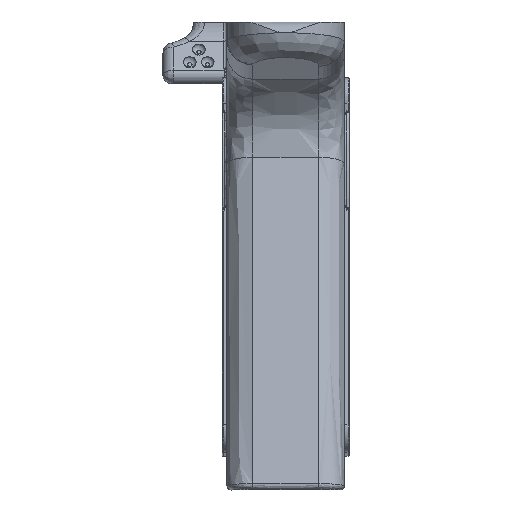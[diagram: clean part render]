
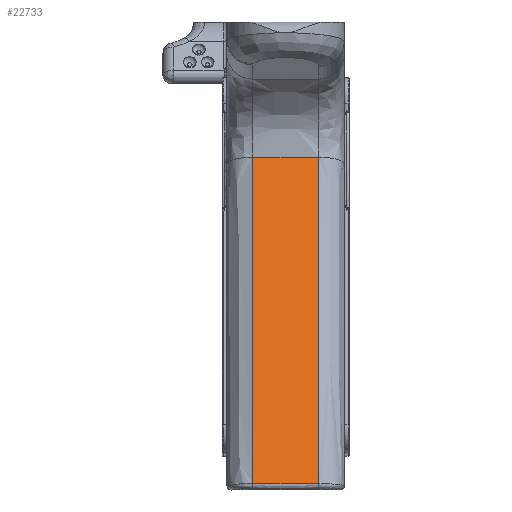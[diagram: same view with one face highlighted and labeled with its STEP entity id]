
A CAD part, front view. The second image highlights one B-rep face of the part: STEP entity #22733.
In plain terms, the highlighted free-form (B-spline) face has degree [5, 1] with [25, 2] control points.
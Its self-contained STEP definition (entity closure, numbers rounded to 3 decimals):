
#752=(
BOUNDED_SURFACE()
B_SPLINE_SURFACE(5,1,((#31762,#31763),(#31764,#31765),(#31766,#31767),(#31768,
#31769),(#31770,#31771),(#31772,#31773),(#31774,#31775),(#31776,#31777),
(#31778,#31779),(#31780,#31781),(#31782,#31783),(#31784,#31785),(#31786,
#31787),(#31788,#31789),(#31790,#31791),(#31792,#31793),(#31794,#31795),
(#31796,#31797),(#31798,#31799),(#31800,#31801),(#31802,#31803),(#31804,
#31805),(#31806,#31807),(#31808,#31809),(#31810,#31811)),.UNSPECIFIED.,
 .F.,.F.,.F.)
B_SPLINE_SURFACE_WITH_KNOTS((6,5,1,1,1,1,1,1,1,1,1,5,6),(2,2),(-1.178,
-1.,-0.9,-0.8,-0.7,-0.6,-0.5,-0.4,-0.3,-0.2,-0.1,0.,2.179),(-2.379,
5.132),.UNSPECIFIED.)
GEOMETRIC_REPRESENTATION_ITEM()
RATIONAL_B_SPLINE_SURFACE(((1.,1.),(1.,1.),(1.,1.),(1.,1.),(1.,1.),(1.,
1.),(1.,1.),(1.,1.),(1.,1.),(1.,1.),(1.,1.),(1.,1.),(1.,1.),(1.,1.),(1.,
1.),(1.,1.),(1.,1.),(1.,1.),(1.,1.),(1.,1.),(1.,1.),(1.,1.),(1.,1.),(1.,
1.),(1.,1.)))
REPRESENTATION_ITEM('')
SURFACE()
);
#1715=B_SPLINE_CURVE_WITH_KNOTS('',3,(#30385,#30386,#30387,#30388,#30389,
#30390),.UNSPECIFIED.,.F.,.F.,(4,2,4),(-7.954,-0.629,
0.),.UNSPECIFIED.);
#1726=B_SPLINE_CURVE_WITH_KNOTS('',3,(#30677,#30678,#30679,#30680,#30681,
#30682,#30683),.UNSPECIFIED.,.F.,.F.,(4,2,1,4),(-7.954,-7.325,
-3.139,0.),.UNSPECIFIED.);
#1804=B_SPLINE_CURVE_WITH_KNOTS('',3,(#31754,#31755,#31756,#31757),
 .UNSPECIFIED.,.F.,.F.,(4,4),(0.6,2.145),.UNSPECIFIED.);
#2730=FACE_OUTER_BOUND('',#4118,.T.);
#4118=EDGE_LOOP('',(#15547,#15548,#15549,#15550));
#5507=LINE('',#30283,#7095);
#7095=VECTOR('',#25575,10.);
#9281=VERTEX_POINT('',#30155);
#9289=VERTEX_POINT('',#30282);
#9291=VERTEX_POINT('',#30384);
#9330=VERTEX_POINT('',#30675);
#11587=EDGE_CURVE('',#9281,#9289,#5507,.T.);
#11591=EDGE_CURVE('',#9289,#9291,#1715,.T.);
#11644=EDGE_CURVE('',#9330,#9281,#1726,.T.);
#11855=EDGE_CURVE('',#9291,#9330,#1804,.T.);
#15547=ORIENTED_EDGE('',*,*,#11591,.F.);
#15548=ORIENTED_EDGE('',*,*,#11587,.F.);
#15549=ORIENTED_EDGE('',*,*,#11644,.F.);
#15550=ORIENTED_EDGE('',*,*,#11855,.F.);
#22733=ADVANCED_FACE('',(#2730),#752,.F.);
#25575=DIRECTION('',(1.,0.,0.));
#30155=CARTESIAN_POINT('',(0.725,-90.162,100.53));
#30282=CARTESIAN_POINT('',(16.175,-90.162,100.53));
#30283=CARTESIAN_POINT('',(22.175,-90.162,100.53));
#30384=CARTESIAN_POINT('',(16.175,-68.765,24.118));
#30385=CARTESIAN_POINT('Ctrl Pts',(16.175,-90.162,100.53));
#30386=CARTESIAN_POINT('Ctrl Pts',(16.175,-83.279,77.132));
#30387=CARTESIAN_POINT('Ctrl Pts',(16.175,-76.502,53.727));
#30388=CARTESIAN_POINT('Ctrl Pts',(16.175,-69.825,28.185));
#30389=CARTESIAN_POINT('Ctrl Pts',(16.175,-69.294,26.148));
#30390=CARTESIAN_POINT('Ctrl Pts',(16.175,-68.765,24.118));
#30675=CARTESIAN_POINT('',(0.725,-68.765,24.118));
#30677=CARTESIAN_POINT('Ctrl Pts',(0.725,-68.765,24.118));
#30678=CARTESIAN_POINT('Ctrl Pts',(0.725,-69.294,
26.148));
#30679=CARTESIAN_POINT('Ctrl Pts',(0.725,-69.824,
28.178));
#30680=CARTESIAN_POINT('Ctrl Pts',(0.725,-73.858,
43.642));
#30681=CARTESIAN_POINT('Ctrl Pts',(0.725,-80.386,
67.092));
#30682=CARTESIAN_POINT('Ctrl Pts',(0.725,-87.212,
90.502));
#30683=CARTESIAN_POINT('Ctrl Pts',(0.725,-90.162,
100.53));
#31754=CARTESIAN_POINT('Ctrl Pts',(16.175,-68.765,24.118));
#31755=CARTESIAN_POINT('Ctrl Pts',(11.025,-68.765,24.118));
#31756=CARTESIAN_POINT('Ctrl Pts',(5.875,-68.765,24.118));
#31757=CARTESIAN_POINT('Ctrl Pts',(0.725,-68.765,24.118));
#31762=CARTESIAN_POINT('Ctrl Pts',(45.968,-95.649,119.15));
#31763=CARTESIAN_POINT('Ctrl Pts',(-29.15,-95.649,
119.15));
#31764=CARTESIAN_POINT('Ctrl Pts',(45.968,-94.719,115.995));
#31765=CARTESIAN_POINT('Ctrl Pts',(-29.15,-94.719,
115.995));
#31766=CARTESIAN_POINT('Ctrl Pts',(45.968,-93.789,112.841));
#31767=CARTESIAN_POINT('Ctrl Pts',(-29.15,-93.789,112.841));
#31768=CARTESIAN_POINT('Ctrl Pts',(45.968,-92.86,109.686));
#31769=CARTESIAN_POINT('Ctrl Pts',(-29.15,-92.86,
109.686));
#31770=CARTESIAN_POINT('Ctrl Pts',(45.968,-91.93,106.531));
#31771=CARTESIAN_POINT('Ctrl Pts',(-29.15,-91.93,
106.531));
#31772=CARTESIAN_POINT('Ctrl Pts',(45.968,-91.,103.376));
#31773=CARTESIAN_POINT('Ctrl Pts',(-29.15,-91.,
103.376));
#31774=CARTESIAN_POINT('Ctrl Pts',(45.968,-90.477,101.6));
#31775=CARTESIAN_POINT('Ctrl Pts',(-29.15,-90.477,
101.6));
#31776=CARTESIAN_POINT('Ctrl Pts',(45.968,-89.439,98.075));
#31777=CARTESIAN_POINT('Ctrl Pts',(-29.15,-89.439,
98.075));
#31778=CARTESIAN_POINT('Ctrl Pts',(45.968,-87.911,92.865));
#31779=CARTESIAN_POINT('Ctrl Pts',(-29.15,-87.911,
92.865));
#31780=CARTESIAN_POINT('Ctrl Pts',(45.968,-85.928,86.075));
#31781=CARTESIAN_POINT('Ctrl Pts',(-29.15,-85.928,
86.075));
#31782=CARTESIAN_POINT('Ctrl Pts',(45.968,-83.55,77.871));
#31783=CARTESIAN_POINT('Ctrl Pts',(-29.15,-83.55,
77.871));
#31784=CARTESIAN_POINT('Ctrl Pts',(45.968,-81.281,69.978));
#31785=CARTESIAN_POINT('Ctrl Pts',(-29.15,-81.281,
69.978));
#31786=CARTESIAN_POINT('Ctrl Pts',(45.968,-79.134,62.429));
#31787=CARTESIAN_POINT('Ctrl Pts',(-29.15,-79.134,
62.429));
#31788=CARTESIAN_POINT('Ctrl Pts',(45.968,-77.12,55.253));
#31789=CARTESIAN_POINT('Ctrl Pts',(-29.15,-77.12,
55.253));
#31790=CARTESIAN_POINT('Ctrl Pts',(45.968,-75.239,48.457));
#31791=CARTESIAN_POINT('Ctrl Pts',(-29.15,-75.239,
48.457));
#31792=CARTESIAN_POINT('Ctrl Pts',(45.968,-73.485,42.019));
#31793=CARTESIAN_POINT('Ctrl Pts',(-29.15,-73.485,
42.019));
#31794=CARTESIAN_POINT('Ctrl Pts',(45.968,-72.177,37.138));
#31795=CARTESIAN_POINT('Ctrl Pts',(-29.15,-72.177,
37.138));
#31796=CARTESIAN_POINT('Ctrl Pts',(45.968,-71.246,33.618));
#31797=CARTESIAN_POINT('Ctrl Pts',(-29.15,-71.246,33.618));
#31798=CARTESIAN_POINT('Ctrl Pts',(45.968,-70.647,31.334));
#31799=CARTESIAN_POINT('Ctrl Pts',(-29.15,-70.647,
31.334));
#31800=CARTESIAN_POINT('Ctrl Pts',(45.968,-70.353,30.208));
#31801=CARTESIAN_POINT('Ctrl Pts',(-29.15,-70.353,
30.208));
#31802=CARTESIAN_POINT('Ctrl Pts',(45.968,-63.949,5.658));
#31803=CARTESIAN_POINT('Ctrl Pts',(-29.15,-63.949,
5.658));
#31804=CARTESIAN_POINT('Ctrl Pts',(45.968,-57.545,-18.892));
#31805=CARTESIAN_POINT('Ctrl Pts',(-29.15,-57.545,
-18.892));
#31806=CARTESIAN_POINT('Ctrl Pts',(45.968,-51.14,-43.442));
#31807=CARTESIAN_POINT('Ctrl Pts',(-29.15,-51.14,
-43.442));
#31808=CARTESIAN_POINT('Ctrl Pts',(45.968,-44.736,-67.992));
#31809=CARTESIAN_POINT('Ctrl Pts',(-29.15,-44.736,
-67.992));
#31810=CARTESIAN_POINT('Ctrl Pts',(45.968,-38.332,-92.542));
#31811=CARTESIAN_POINT('Ctrl Pts',(-29.15,-38.332,-92.542));
